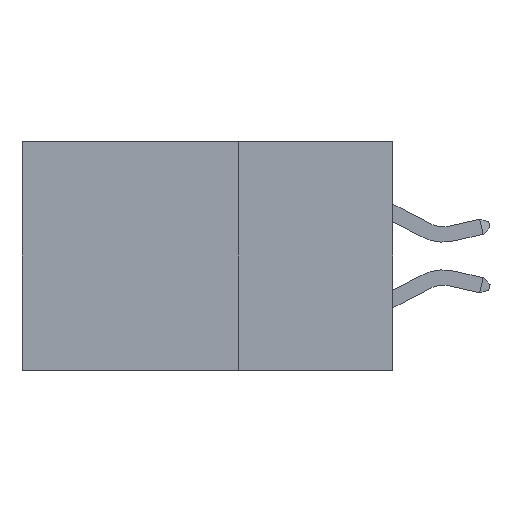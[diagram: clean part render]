
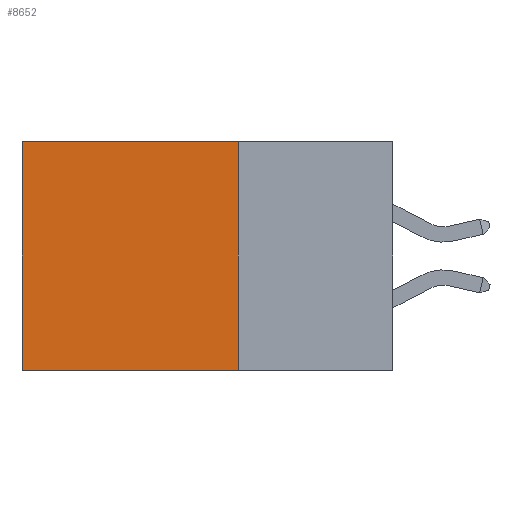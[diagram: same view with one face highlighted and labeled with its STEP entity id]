
A CAD part, left-side view. The second image highlights one B-rep face of the part: STEP entity #8652.
In plain terms, the highlighted planar face has unit normal (-1, 0, 0).
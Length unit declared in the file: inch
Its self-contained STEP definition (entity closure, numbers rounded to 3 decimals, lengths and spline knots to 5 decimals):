
#316 = PLANE ( 'NONE',  #16471 ) ;
#662 = CARTESIAN_POINT ( 'NONE',  ( 0.2875, 0.6, -0.37 ) ) ;
#747 = CARTESIAN_POINT ( 'NONE',  ( 0.2875, 0.6, 0. ) ) ;
#821 = FACE_OUTER_BOUND ( 'NONE', #12365, .T. ) ;
#2056 = DIRECTION ( 'NONE',  ( 0., 0., -1. ) ) ;
#3093 = VECTOR ( 'NONE', #3759, 39.37008 ) ;
#3367 = VERTEX_POINT ( 'NONE', #13367 ) ;
#3759 = DIRECTION ( 'NONE',  ( 0., 0., -1. ) ) ;
#3998 = EDGE_CURVE ( 'NONE', #14437, #6562, #5187, .T. ) ;
#4277 = LINE ( 'NONE', #16217, #11278 ) ;
#5187 = LINE ( 'NONE', #747, #3093 ) ;
#5268 = ORIENTED_EDGE ( 'NONE', *, *, #3998, .T. ) ;
#5579 = DIRECTION ( 'NONE',  ( 0., 1., 0. ) ) ;
#6562 = VERTEX_POINT ( 'NONE', #662 ) ;
#6676 = CARTESIAN_POINT ( 'NONE',  ( 0.2875, 0.25, 0. ) ) ;
#7125 = CARTESIAN_POINT ( 'NONE',  ( 0.2875, 0.6, 0. ) ) ;
#7137 = LINE ( 'NONE', #7463, #18133 ) ;
#7463 = CARTESIAN_POINT ( 'NONE',  ( 0.2875, 0.25, 0. ) ) ;
#7746 = ORIENTED_EDGE ( 'NONE', *, *, #8899, .T. ) ;
#8652 = ADVANCED_FACE ( 'NONE', ( #821 ), #316, .F. ) ;
#8899 = EDGE_CURVE ( 'NONE', #3367, #14437, #7137, .T. ) ;
#10662 = ORIENTED_EDGE ( 'NONE', *, *, #19276, .F. ) ;
#11278 = VECTOR ( 'NONE', #19296, 39.37008 ) ;
#11508 = CARTESIAN_POINT ( 'NONE',  ( 0.2875, 0.25, -0.37 ) ) ;
#11994 = CARTESIAN_POINT ( 'NONE',  ( 0.2875, 0.25, -0.37 ) ) ;
#12365 = EDGE_LOOP ( 'NONE', ( #5268, #10662, #15387, #7746 ) ) ;
#13367 = CARTESIAN_POINT ( 'NONE',  ( 0.2875, 0.25, 0. ) ) ;
#13529 = EDGE_CURVE ( 'NONE', #3367, #18843, #4277, .T. ) ;
#13792 = VECTOR ( 'NONE', #5579, 39.37008 ) ;
#14437 = VERTEX_POINT ( 'NONE', #7125 ) ;
#15387 = ORIENTED_EDGE ( 'NONE', *, *, #13529, .F. ) ;
#16217 = CARTESIAN_POINT ( 'NONE',  ( 0.2875, 0.25, 0. ) ) ;
#16471 = AXIS2_PLACEMENT_3D ( 'NONE', #6676, #17092, #2056 ) ;
#16616 = LINE ( 'NONE', #11508, #13792 ) ;
#17092 = DIRECTION ( 'NONE',  ( 1., 0., 0. ) ) ;
#18058 = DIRECTION ( 'NONE',  ( 0., 1., 0. ) ) ;
#18133 = VECTOR ( 'NONE', #18058, 39.37008 ) ;
#18843 = VERTEX_POINT ( 'NONE', #11994 ) ;
#19276 = EDGE_CURVE ( 'NONE', #18843, #6562, #16616, .T. ) ;
#19296 = DIRECTION ( 'NONE',  ( 0., 0., -1. ) ) ;
